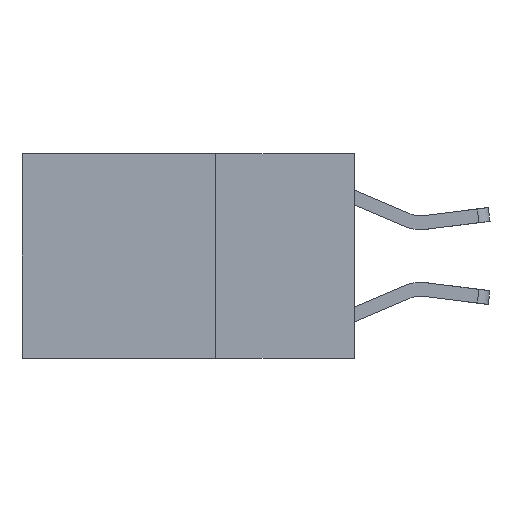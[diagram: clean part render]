
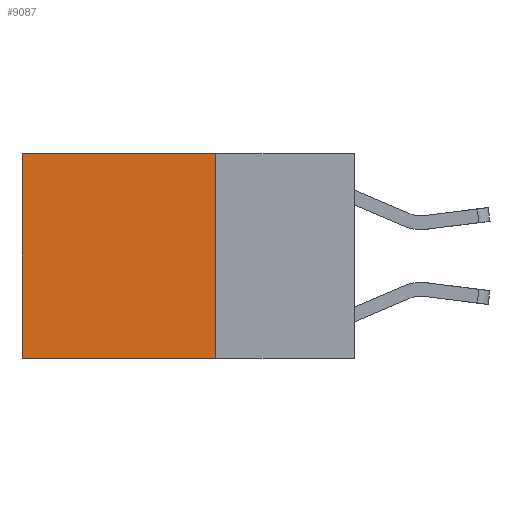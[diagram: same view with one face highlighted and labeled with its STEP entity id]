
A CAD part, left-side view. The second image highlights one B-rep face of the part: STEP entity #9087.
In plain terms, the highlighted planar face has unit normal (-1, 0, 0).
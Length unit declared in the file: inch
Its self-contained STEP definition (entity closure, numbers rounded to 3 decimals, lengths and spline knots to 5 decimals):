
#148 = ORIENTED_EDGE ( 'NONE', *, *, #2445, .T. ) ;
#295 = EDGE_CURVE ( 'NONE', #2380, #6257, #3803, .T. ) ;
#571 = LINE ( 'NONE', #4380, #9068 ) ;
#775 = VECTOR ( 'NONE', #2052, 39.37008 ) ;
#1064 = CARTESIAN_POINT ( 'NONE',  ( 0.2625, 0.6, -0.37 ) ) ;
#2052 = DIRECTION ( 'NONE',  ( 0., 1., 0. ) ) ;
#2081 = ORIENTED_EDGE ( 'NONE', *, *, #8085, .F. ) ;
#2297 = CARTESIAN_POINT ( 'NONE',  ( 0.2625, 0.6, 0. ) ) ;
#2380 = VERTEX_POINT ( 'NONE', #3046 ) ;
#2445 = EDGE_CURVE ( 'NONE', #5910, #6218, #9334, .T. ) ;
#2904 = CARTESIAN_POINT ( 'NONE',  ( 0.2625, 0.25, -0.37 ) ) ;
#3046 = CARTESIAN_POINT ( 'NONE',  ( 0.2625, 0.25, 0. ) ) ;
#3292 = LINE ( 'NONE', #2904, #775 ) ;
#3392 = DIRECTION ( 'NONE',  ( 0., 0., -1. ) ) ;
#3803 = LINE ( 'NONE', #9645, #8385 ) ;
#3912 = EDGE_CURVE ( 'NONE', #2380, #5910, #571, .T. ) ;
#3982 = CARTESIAN_POINT ( 'NONE',  ( 0.2625, 0.6, 0. ) ) ;
#4380 = CARTESIAN_POINT ( 'NONE',  ( 0.2625, 0.25, 0. ) ) ;
#4460 = CARTESIAN_POINT ( 'NONE',  ( 0.2625, 0.25, -0.37 ) ) ;
#4781 = DIRECTION ( 'NONE',  ( 0., 0., -1. ) ) ;
#5216 = DIRECTION ( 'NONE',  ( 0., 1., 0. ) ) ;
#5531 = AXIS2_PLACEMENT_3D ( 'NONE', #7449, #8272, #3392 ) ;
#5656 = EDGE_LOOP ( 'NONE', ( #148, #2081, #5792, #8730 ) ) ;
#5792 = ORIENTED_EDGE ( 'NONE', *, *, #295, .F. ) ;
#5851 = PLANE ( 'NONE',  #5531 ) ;
#5910 = VERTEX_POINT ( 'NONE', #3982 ) ;
#6218 = VERTEX_POINT ( 'NONE', #1064 ) ;
#6257 = VERTEX_POINT ( 'NONE', #4460 ) ;
#7449 = CARTESIAN_POINT ( 'NONE',  ( 0.2625, 0.25, 0. ) ) ;
#7698 = VECTOR ( 'NONE', #4781, 39.37008 ) ;
#8085 = EDGE_CURVE ( 'NONE', #6257, #6218, #3292, .T. ) ;
#8272 = DIRECTION ( 'NONE',  ( 1., 0., 0. ) ) ;
#8385 = VECTOR ( 'NONE', #8837, 39.37008 ) ;
#8730 = ORIENTED_EDGE ( 'NONE', *, *, #3912, .T. ) ;
#8837 = DIRECTION ( 'NONE',  ( 0., 0., -1. ) ) ;
#9068 = VECTOR ( 'NONE', #5216, 39.37008 ) ;
#9087 = ADVANCED_FACE ( 'NONE', ( #10636 ), #5851, .F. ) ;
#9334 = LINE ( 'NONE', #2297, #7698 ) ;
#9645 = CARTESIAN_POINT ( 'NONE',  ( 0.2625, 0.25, 0. ) ) ;
#10636 = FACE_OUTER_BOUND ( 'NONE', #5656, .T. ) ;
